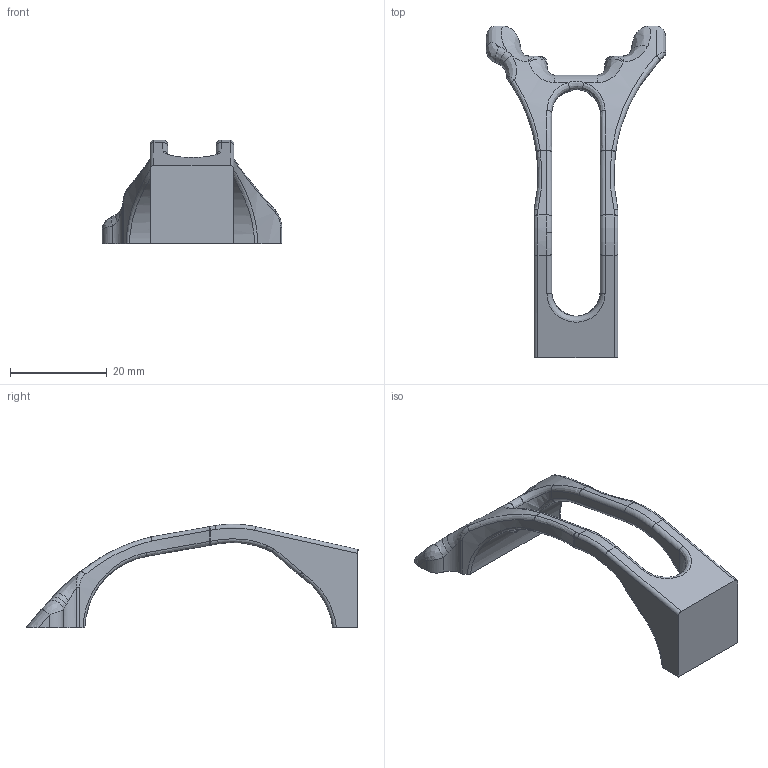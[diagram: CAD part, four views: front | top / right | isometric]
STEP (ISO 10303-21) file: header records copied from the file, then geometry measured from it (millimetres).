
FILE_DESCRIPTION (( 'STEP AP214' ), '1' );
FILE_NAME ('4.STEP', '2013-09-29T07:11:41', ( 'elpi' ), ( '' ), 'SwSTEP 2.0', 'SolidWorks 2013', '' );
FILE_SCHEMA (( 'AUTOMOTIVE_DESIGN' ));
Length unit declared in the file: millimetre
Products named in the file (1): 4
Bounding box: 37.13 x 68.55 x 21.44 mm (x, y, z)
Volume: 5920.7 mm3; surface area: 3746.7 mm2
Topology: 1 solids, 1 shells, 141 faces, 341 edges, 196 vertices
Faces by surface type: bspline 51, cylinder 45, plane 23, torus 16, sphere 6
Entity records: 6269 total; most frequent: CARTESIAN_POINT 3357, ORIENTED_EDGE 674, DIRECTION 511, EDGE_CURVE 337, AXIS2_PLACEMENT_3D 201, VERTEX_POINT 196, EDGE_LOOP 141, FACE_OUTER_BOUND 141
